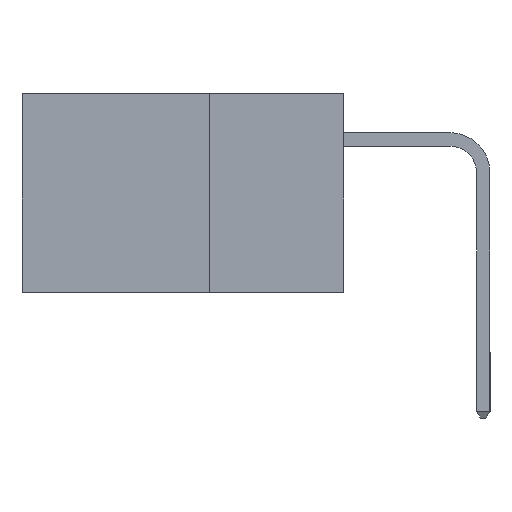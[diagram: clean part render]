
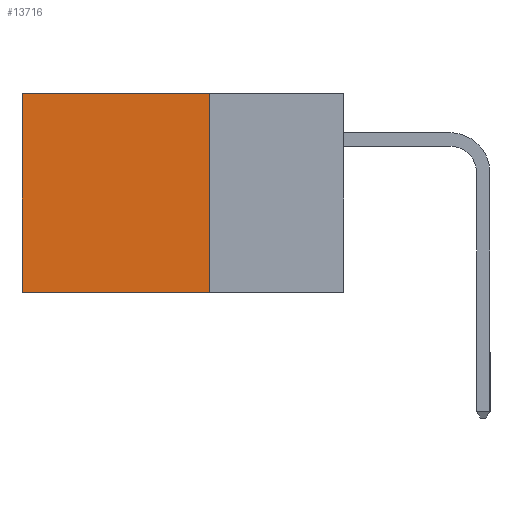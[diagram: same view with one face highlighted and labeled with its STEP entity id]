
A CAD part, left-side view. The second image highlights one B-rep face of the part: STEP entity #13716.
In plain terms, the highlighted planar face has unit normal (-1, 0, 0).
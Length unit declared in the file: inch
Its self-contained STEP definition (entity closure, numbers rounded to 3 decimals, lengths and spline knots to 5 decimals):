
#63 = CARTESIAN_POINT ( 'NONE',  ( 0.298, 0.6, 0. ) ) ;
#633 = CARTESIAN_POINT ( 'NONE',  ( 0.298, 0.25, -0.37 ) ) ;
#1706 = EDGE_LOOP ( 'NONE', ( #17483, #30583, #17599, #7318 ) ) ;
#2456 = VECTOR ( 'NONE', #29050, 39.37008 ) ;
#3859 = VERTEX_POINT ( 'NONE', #11175 ) ;
#5776 = LINE ( 'NONE', #63, #30542 ) ;
#5949 = CARTESIAN_POINT ( 'NONE',  ( 0.298, 0.6, 0. ) ) ;
#7318 = ORIENTED_EDGE ( 'NONE', *, *, #23612, .T. ) ;
#8213 = DIRECTION ( 'NONE',  ( 1., 0., 0. ) ) ;
#8525 = DIRECTION ( 'NONE',  ( 0., 0., -1. ) ) ;
#11175 = CARTESIAN_POINT ( 'NONE',  ( 0.298, 0.25, 0. ) ) ;
#11247 = CARTESIAN_POINT ( 'NONE',  ( 0.298, 0.25, 0. ) ) ;
#12004 = VECTOR ( 'NONE', #14730, 39.37008 ) ;
#12623 = CARTESIAN_POINT ( 'NONE',  ( 0.298, 0.25, 0. ) ) ;
#13716 = ADVANCED_FACE ( 'NONE', ( #19938 ), #22720, .F. ) ;
#14301 = CARTESIAN_POINT ( 'NONE',  ( 0.298, 0.6, -0.37 ) ) ;
#14730 = DIRECTION ( 'NONE',  ( 0., 1., 0. ) ) ;
#16161 = LINE ( 'NONE', #12623, #2456 ) ;
#17483 = ORIENTED_EDGE ( 'NONE', *, *, #22496, .T. ) ;
#17599 = ORIENTED_EDGE ( 'NONE', *, *, #22143, .F. ) ;
#17997 = CARTESIAN_POINT ( 'NONE',  ( 0.298, 0.25, 0. ) ) ;
#18278 = LINE ( 'NONE', #633, #12004 ) ;
#18684 = DIRECTION ( 'NONE',  ( 0., 0., -1. ) ) ;
#19938 = FACE_OUTER_BOUND ( 'NONE', #1706, .T. ) ;
#20135 = VERTEX_POINT ( 'NONE', #21874 ) ;
#20362 = VERTEX_POINT ( 'NONE', #5949 ) ;
#21874 = CARTESIAN_POINT ( 'NONE',  ( 0.298, 0.25, -0.37 ) ) ;
#21965 = VECTOR ( 'NONE', #30461, 39.37008 ) ;
#22143 = EDGE_CURVE ( 'NONE', #3859, #20135, #16161, .T. ) ;
#22496 = EDGE_CURVE ( 'NONE', #20362, #25302, #5776, .T. ) ;
#22720 = PLANE ( 'NONE',  #29169 ) ;
#23242 = EDGE_CURVE ( 'NONE', #20135, #25302, #18278, .T. ) ;
#23612 = EDGE_CURVE ( 'NONE', #3859, #20362, #27147, .T. ) ;
#25302 = VERTEX_POINT ( 'NONE', #14301 ) ;
#27147 = LINE ( 'NONE', #11247, #21965 ) ;
#29050 = DIRECTION ( 'NONE',  ( 0., 0., -1. ) ) ;
#29169 = AXIS2_PLACEMENT_3D ( 'NONE', #17997, #8213, #8525 ) ;
#30461 = DIRECTION ( 'NONE',  ( 0., 1., 0. ) ) ;
#30542 = VECTOR ( 'NONE', #18684, 39.37008 ) ;
#30583 = ORIENTED_EDGE ( 'NONE', *, *, #23242, .F. ) ;
